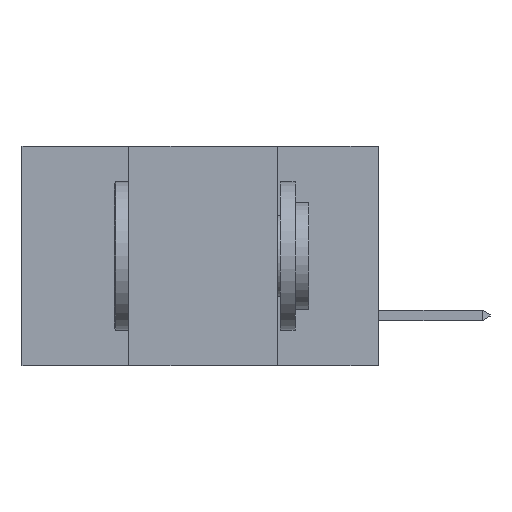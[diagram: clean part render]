
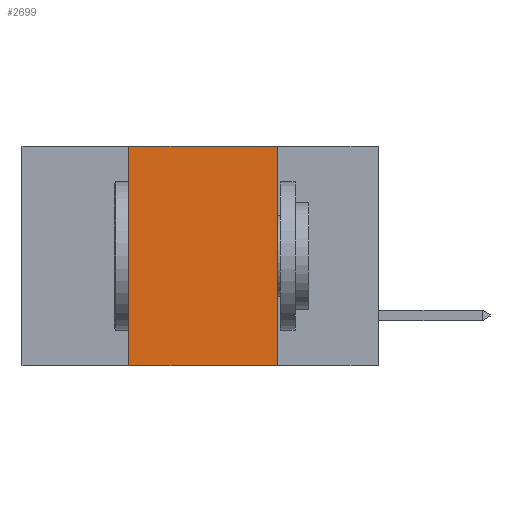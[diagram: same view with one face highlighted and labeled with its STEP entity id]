
A CAD part, left-side view. The second image highlights one B-rep face of the part: STEP entity #2699.
In plain terms, the highlighted planar face has unit normal (-1, 0, 0).
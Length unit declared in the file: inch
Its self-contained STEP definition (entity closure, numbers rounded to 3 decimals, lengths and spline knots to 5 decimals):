
#208 = FACE_OUTER_BOUND ( 'NONE', #672, .T. ) ;
#606 = EDGE_CURVE ( 'NONE', #10859, #2855, #1418, .T. ) ;
#637 = CARTESIAN_POINT ( 'NONE',  ( 0., 0.42, -0.37 ) ) ;
#666 = CARTESIAN_POINT ( 'NONE',  ( 0., 0.17, 0. ) ) ;
#672 = EDGE_LOOP ( 'NONE', ( #9053, #8900, #8899, #8889 ) ) ;
#1181 = VERTEX_POINT ( 'NONE', #666 ) ;
#1418 = LINE ( 'NONE', #7166, #6002 ) ;
#1639 = LINE ( 'NONE', #10272, #6164 ) ;
#2699 = ADVANCED_FACE ( 'NONE', ( #208 ), #10111, .F. ) ;
#2855 = VERTEX_POINT ( 'NONE', #8096 ) ;
#3015 = DIRECTION ( 'NONE',  ( 0., -1., 0. ) ) ;
#4149 = EDGE_CURVE ( 'NONE', #1181, #5795, #1639, .T. ) ;
#4818 = VECTOR ( 'NONE', #3015, 39.37008 ) ;
#4836 = CARTESIAN_POINT ( 'NONE',  ( 0., 0.6, 0. ) ) ;
#4876 = AXIS2_PLACEMENT_3D ( 'NONE', #10211, #10101, #10058 ) ;
#5691 = LINE ( 'NONE', #7891, #7662 ) ;
#5795 = VERTEX_POINT ( 'NONE', #6987 ) ;
#6002 = VECTOR ( 'NONE', #9469, 39.37008 ) ;
#6164 = VECTOR ( 'NONE', #10295, 39.37008 ) ;
#6987 = CARTESIAN_POINT ( 'NONE',  ( 0., 0.17, -0.37 ) ) ;
#7166 = CARTESIAN_POINT ( 'NONE',  ( 0., 0.42, -0.37 ) ) ;
#7285 = LINE ( 'NONE', #4836, #4818 ) ;
#7335 = EDGE_CURVE ( 'NONE', #2855, #1181, #7285, .T. ) ;
#7662 = VECTOR ( 'NONE', #10533, 39.37008 ) ;
#7891 = CARTESIAN_POINT ( 'NONE',  ( 0., 0.6, -0.37 ) ) ;
#8096 = CARTESIAN_POINT ( 'NONE',  ( 0., 0.42, 0. ) ) ;
#8889 = ORIENTED_EDGE ( 'NONE', *, *, #10736, .T. ) ;
#8899 = ORIENTED_EDGE ( 'NONE', *, *, #606, .F. ) ;
#8900 = ORIENTED_EDGE ( 'NONE', *, *, #7335, .F. ) ;
#9053 = ORIENTED_EDGE ( 'NONE', *, *, #4149, .F. ) ;
#9469 = DIRECTION ( 'NONE',  ( 0., 0., 1. ) ) ;
#10058 = DIRECTION ( 'NONE',  ( 0., 0., -1. ) ) ;
#10101 = DIRECTION ( 'NONE',  ( 1., 0., 0. ) ) ;
#10111 = PLANE ( 'NONE',  #4876 ) ;
#10211 = CARTESIAN_POINT ( 'NONE',  ( 0., 0.6, 0. ) ) ;
#10272 = CARTESIAN_POINT ( 'NONE',  ( 0., 0.17, -0.37 ) ) ;
#10295 = DIRECTION ( 'NONE',  ( 0., 0., -1. ) ) ;
#10533 = DIRECTION ( 'NONE',  ( 0., -1., 0. ) ) ;
#10736 = EDGE_CURVE ( 'NONE', #10859, #5795, #5691, .T. ) ;
#10859 = VERTEX_POINT ( 'NONE', #637 ) ;
